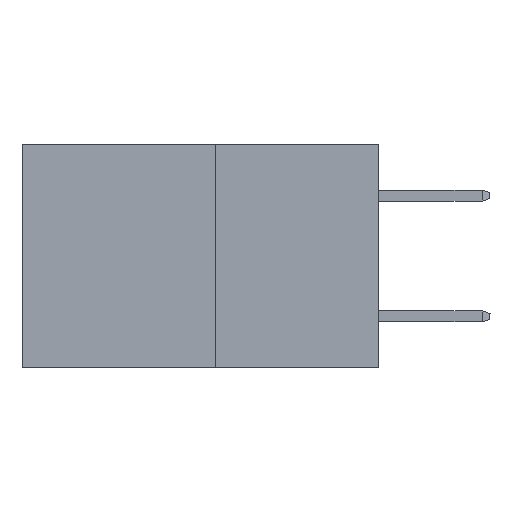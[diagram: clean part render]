
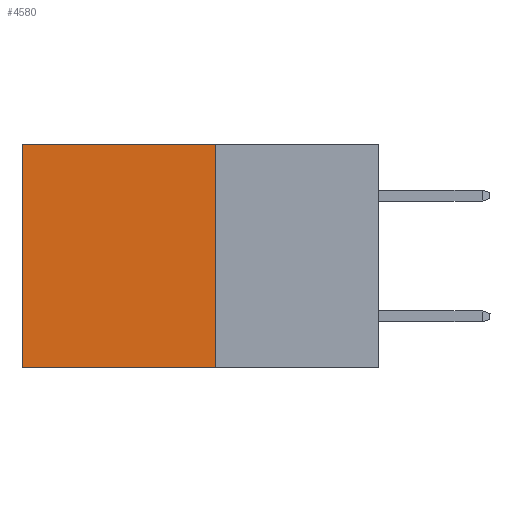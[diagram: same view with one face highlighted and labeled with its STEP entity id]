
A CAD part, left-side view. The second image highlights one B-rep face of the part: STEP entity #4580.
In plain terms, the highlighted planar face has unit normal (-1, 0, 0).
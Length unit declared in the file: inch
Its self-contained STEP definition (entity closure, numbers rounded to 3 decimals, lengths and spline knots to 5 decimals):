
#189 = EDGE_CURVE ( 'NONE', #9028, #4708, #2167, .T. ) ;
#196 = ORIENTED_EDGE ( 'NONE', *, *, #6133, .F. ) ;
#1053 = VERTEX_POINT ( 'NONE', #4367 ) ;
#1392 = CARTESIAN_POINT ( 'NONE',  ( 0.277, 0.27, 0. ) ) ;
#1937 = EDGE_CURVE ( 'NONE', #9028, #1053, #10033, .T. ) ;
#2167 = LINE ( 'NONE', #6708, #11183 ) ;
#2347 = DIRECTION ( 'NONE',  ( 0., 1., 0. ) ) ;
#2355 = LINE ( 'NONE', #7764, #6956 ) ;
#3314 = EDGE_CURVE ( 'NONE', #1053, #3682, #8308, .T. ) ;
#3634 = EDGE_LOOP ( 'NONE', ( #10008, #196, #4285, #3970 ) ) ;
#3682 = VERTEX_POINT ( 'NONE', #8937 ) ;
#3970 = ORIENTED_EDGE ( 'NONE', *, *, #1937, .T. ) ;
#4096 = DIRECTION ( 'NONE',  ( 1., 0., 0. ) ) ;
#4248 = CARTESIAN_POINT ( 'NONE',  ( 0.277, 0.27, -0.37 ) ) ;
#4285 = ORIENTED_EDGE ( 'NONE', *, *, #189, .F. ) ;
#4367 = CARTESIAN_POINT ( 'NONE',  ( 0.277, 0.59, 0. ) ) ;
#4580 = ADVANCED_FACE ( 'NONE', ( #7370 ), #9254, .F. ) ;
#4708 = VERTEX_POINT ( 'NONE', #4248 ) ;
#5091 = CARTESIAN_POINT ( 'NONE',  ( 0.277, 0.59, -0.37 ) ) ;
#5575 = VECTOR ( 'NONE', #7008, 39.37008 ) ;
#6133 = EDGE_CURVE ( 'NONE', #4708, #3682, #2355, .T. ) ;
#6484 = AXIS2_PLACEMENT_3D ( 'NONE', #6723, #4096, #10066 ) ;
#6708 = CARTESIAN_POINT ( 'NONE',  ( 0.277, 0.27, -0.37 ) ) ;
#6723 = CARTESIAN_POINT ( 'NONE',  ( 0.277, 0.27, -0.37 ) ) ;
#6956 = VECTOR ( 'NONE', #2347, 39.37008 ) ;
#7008 = DIRECTION ( 'NONE',  ( 0., 1., 0. ) ) ;
#7370 = FACE_OUTER_BOUND ( 'NONE', #3634, .T. ) ;
#7764 = CARTESIAN_POINT ( 'NONE',  ( 0.277, 0.27, -0.37 ) ) ;
#7796 = CARTESIAN_POINT ( 'NONE',  ( 0.277, 0.27, 0. ) ) ;
#8308 = LINE ( 'NONE', #5091, #10753 ) ;
#8937 = CARTESIAN_POINT ( 'NONE',  ( 0.277, 0.59, -0.37 ) ) ;
#8985 = DIRECTION ( 'NONE',  ( 0., 0., -1. ) ) ;
#9028 = VERTEX_POINT ( 'NONE', #7796 ) ;
#9254 = PLANE ( 'NONE',  #6484 ) ;
#10008 = ORIENTED_EDGE ( 'NONE', *, *, #3314, .T. ) ;
#10033 = LINE ( 'NONE', #1392, #5575 ) ;
#10066 = DIRECTION ( 'NONE',  ( 0., 0., -1. ) ) ;
#10753 = VECTOR ( 'NONE', #10931, 39.37008 ) ;
#10931 = DIRECTION ( 'NONE',  ( 0., 0., -1. ) ) ;
#11183 = VECTOR ( 'NONE', #8985, 39.37008 ) ;
